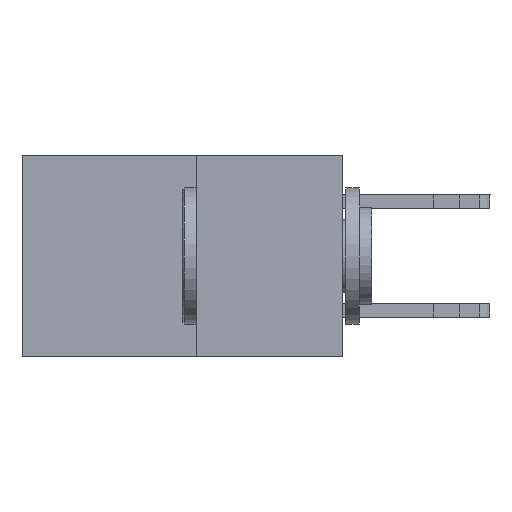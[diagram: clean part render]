
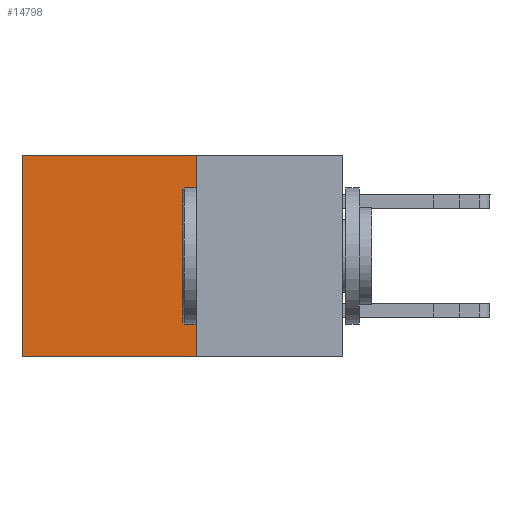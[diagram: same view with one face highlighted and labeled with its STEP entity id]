
A CAD part, left-side view. The second image highlights one B-rep face of the part: STEP entity #14798.
In plain terms, the highlighted planar face has unit normal (-1, 0, 0).
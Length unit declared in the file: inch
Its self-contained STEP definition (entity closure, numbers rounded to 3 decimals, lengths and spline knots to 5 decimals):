
#556 = VECTOR ( 'NONE', #8994, 39.37008 ) ;
#692 = DIRECTION ( 'NONE',  ( 0., 0., -1. ) ) ;
#854 = DIRECTION ( 'NONE',  ( 0., 0., -1. ) ) ;
#1808 = EDGE_LOOP ( 'NONE', ( #9422, #18003, #14578, #11492 ) ) ;
#2467 = CARTESIAN_POINT ( 'NONE',  ( 0.277, 0.27, -0.37 ) ) ;
#2580 = CARTESIAN_POINT ( 'NONE',  ( 0.277, 0.59, -0.37 ) ) ;
#2690 = EDGE_CURVE ( 'NONE', #12755, #8364, #19370, .T. ) ;
#4100 = DIRECTION ( 'NONE',  ( 0., 0., -1. ) ) ;
#5759 = LINE ( 'NONE', #12791, #556 ) ;
#5978 = CARTESIAN_POINT ( 'NONE',  ( 0.277, 0.59, -0.37 ) ) ;
#6334 = AXIS2_PLACEMENT_3D ( 'NONE', #2467, #15643, #854 ) ;
#7259 = LINE ( 'NONE', #15489, #13655 ) ;
#8328 = CARTESIAN_POINT ( 'NONE',  ( 0.277, 0.27, -0.37 ) ) ;
#8364 = VERTEX_POINT ( 'NONE', #5978 ) ;
#8755 = VERTEX_POINT ( 'NONE', #18791 ) ;
#8927 = CARTESIAN_POINT ( 'NONE',  ( 0.277, 0.27, 0. ) ) ;
#8994 = DIRECTION ( 'NONE',  ( 0., 1., 0. ) ) ;
#9422 = ORIENTED_EDGE ( 'NONE', *, *, #19871, .T. ) ;
#10259 = FACE_OUTER_BOUND ( 'NONE', #1808, .T. ) ;
#11492 = ORIENTED_EDGE ( 'NONE', *, *, #17448, .T. ) ;
#12116 = LINE ( 'NONE', #2580, #15659 ) ;
#12755 = VERTEX_POINT ( 'NONE', #8328 ) ;
#12791 = CARTESIAN_POINT ( 'NONE',  ( 0.277, 0.27, 0. ) ) ;
#13655 = VECTOR ( 'NONE', #692, 39.37008 ) ;
#14578 = ORIENTED_EDGE ( 'NONE', *, *, #17276, .F. ) ;
#14798 = ADVANCED_FACE ( 'NONE', ( #10259 ), #16849, .F. ) ;
#15489 = CARTESIAN_POINT ( 'NONE',  ( 0.277, 0.27, -0.37 ) ) ;
#15643 = DIRECTION ( 'NONE',  ( 1., 0., 0. ) ) ;
#15659 = VECTOR ( 'NONE', #4100, 39.37008 ) ;
#16110 = VERTEX_POINT ( 'NONE', #8927 ) ;
#16849 = PLANE ( 'NONE',  #6334 ) ;
#17276 = EDGE_CURVE ( 'NONE', #16110, #12755, #7259, .T. ) ;
#17417 = DIRECTION ( 'NONE',  ( 0., 1., 0. ) ) ;
#17448 = EDGE_CURVE ( 'NONE', #16110, #8755, #5759, .T. ) ;
#18003 = ORIENTED_EDGE ( 'NONE', *, *, #2690, .F. ) ;
#18791 = CARTESIAN_POINT ( 'NONE',  ( 0.277, 0.59, 0. ) ) ;
#19047 = CARTESIAN_POINT ( 'NONE',  ( 0.277, 0.27, -0.37 ) ) ;
#19370 = LINE ( 'NONE', #19047, #20703 ) ;
#19871 = EDGE_CURVE ( 'NONE', #8755, #8364, #12116, .T. ) ;
#20703 = VECTOR ( 'NONE', #17417, 39.37008 ) ;
